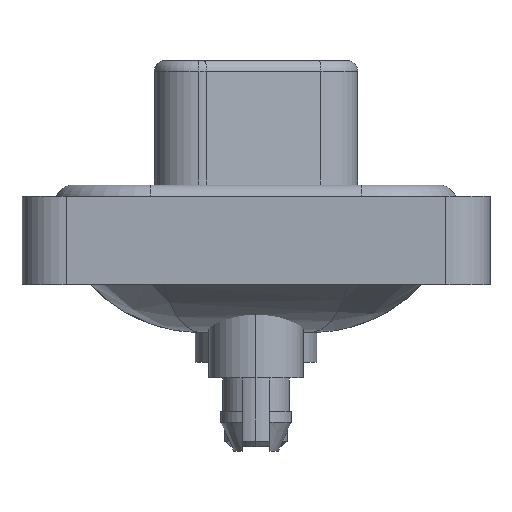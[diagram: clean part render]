
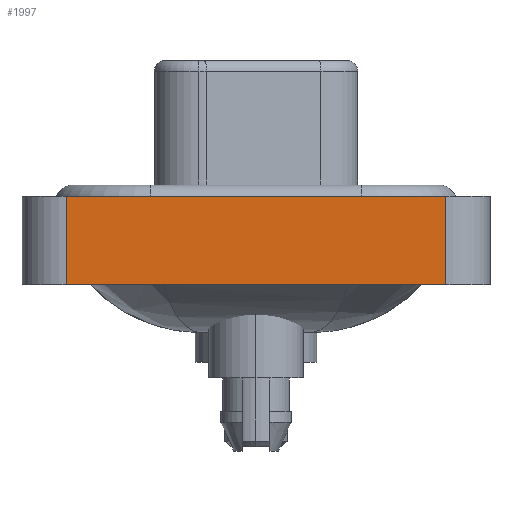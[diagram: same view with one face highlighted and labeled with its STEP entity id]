
A CAD part, left-side view. The second image highlights one B-rep face of the part: STEP entity #1997.
In plain terms, the highlighted planar face has unit normal (-1, 0, 0).
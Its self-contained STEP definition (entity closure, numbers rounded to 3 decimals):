
#505 = LINE ( 'NONE', #7778, #8702 ) ;
#819 = DIRECTION ( 'NONE',  ( 0., 0., 1. ) ) ;
#1185 = EDGE_CURVE ( 'NONE', #10933, #20174, #14404, .T. ) ;
#1197 = ORIENTED_EDGE ( 'NONE', *, *, #7546, .T. ) ;
#1303 = DIRECTION ( 'NONE',  ( 0., 0., 1. ) ) ;
#1997 = ADVANCED_FACE ( 'NONE', ( #18889 ), #22224, .T. ) ;
#2161 = CARTESIAN_POINT ( 'NONE',  ( -7.25, -8.55, 0.4 ) ) ;
#2381 = VERTEX_POINT ( 'NONE', #9881 ) ;
#2746 = AXIS2_PLACEMENT_3D ( 'NONE', #18446, #16598, #819 ) ;
#2898 = VECTOR ( 'NONE', #12649, 1000. ) ;
#3038 = LINE ( 'NONE', #10067, #12081 ) ;
#4425 = EDGE_CURVE ( 'NONE', #10042, #2381, #505, .T. ) ;
#4667 = CARTESIAN_POINT ( 'NONE',  ( -7.25, 8.55, -3.6 ) ) ;
#5642 = CARTESIAN_POINT ( 'NONE',  ( -7.25, -8.55, 0.4 ) ) ;
#7546 = EDGE_CURVE ( 'NONE', #2381, #20174, #3038, .T. ) ;
#7778 = CARTESIAN_POINT ( 'NONE',  ( -7.25, -8.55, -3.6 ) ) ;
#8702 = VECTOR ( 'NONE', #12834, 1000. ) ;
#9438 = CARTESIAN_POINT ( 'NONE',  ( -7.25, 8.55, -3.6 ) ) ;
#9881 = CARTESIAN_POINT ( 'NONE',  ( -7.25, -8.55, -3.6 ) ) ;
#10042 = VERTEX_POINT ( 'NONE', #4667 ) ;
#10067 = CARTESIAN_POINT ( 'NONE',  ( -7.25, -8.55, -3.6 ) ) ;
#10933 = VERTEX_POINT ( 'NONE', #13629 ) ;
#11423 = DIRECTION ( 'NONE',  ( 0., -1., 0. ) ) ;
#11479 = ORIENTED_EDGE ( 'NONE', *, *, #4425, .T. ) ;
#12081 = VECTOR ( 'NONE', #1303, 1000. ) ;
#12649 = DIRECTION ( 'NONE',  ( 0., 0., 1. ) ) ;
#12834 = DIRECTION ( 'NONE',  ( 0., -1., 0. ) ) ;
#13629 = CARTESIAN_POINT ( 'NONE',  ( -7.25, 8.55, 0.4 ) ) ;
#14404 = LINE ( 'NONE', #5642, #16328 ) ;
#15368 = ORIENTED_EDGE ( 'NONE', *, *, #1185, .F. ) ;
#16328 = VECTOR ( 'NONE', #11423, 1000. ) ;
#16577 = LINE ( 'NONE', #9438, #2898 ) ;
#16598 = DIRECTION ( 'NONE',  ( -1., 0., 0. ) ) ;
#18446 = CARTESIAN_POINT ( 'NONE',  ( -7.25, -8.55, -3.6 ) ) ;
#18654 = EDGE_CURVE ( 'NONE', #10042, #10933, #16577, .T. ) ;
#18722 = ORIENTED_EDGE ( 'NONE', *, *, #18654, .F. ) ;
#18889 = FACE_OUTER_BOUND ( 'NONE', #19194, .T. ) ;
#19194 = EDGE_LOOP ( 'NONE', ( #1197, #15368, #18722, #11479 ) ) ;
#20174 = VERTEX_POINT ( 'NONE', #2161 ) ;
#22224 = PLANE ( 'NONE',  #2746 ) ;
